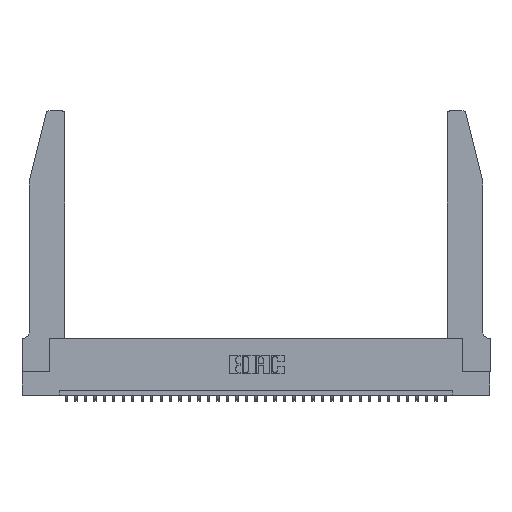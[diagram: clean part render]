
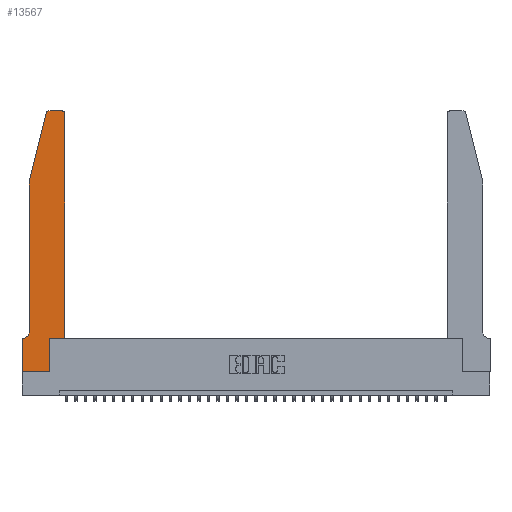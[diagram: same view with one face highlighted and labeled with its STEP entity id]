
A CAD part, top view. The second image highlights one B-rep face of the part: STEP entity #13567.
In plain terms, the highlighted planar face has unit normal (0, 0, 1).
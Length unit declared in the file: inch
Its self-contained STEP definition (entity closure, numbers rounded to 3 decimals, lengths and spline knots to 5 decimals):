
#1578 = CIRCLE ( 'NONE', #30571, 0.07 ) ;
#1940 = VERTEX_POINT ( 'NONE', #26378 ) ;
#2001 = VECTOR ( 'NONE', #25602, 39.37008 ) ;
#2040 = DIRECTION ( 'NONE',  ( -1., 0., 0. ) ) ;
#3359 = CARTESIAN_POINT ( 'NONE',  ( 0.0755, 0.35, 0.37 ) ) ;
#3652 = CARTESIAN_POINT ( 'NONE',  ( 0.0755, 2., 0.37 ) ) ;
#4504 = VERTEX_POINT ( 'NONE', #26337 ) ;
#4756 = FACE_OUTER_BOUND ( 'NONE', #33299, .T. ) ;
#4807 = DIRECTION ( 'NONE',  ( 0., -1., 0. ) ) ;
#4851 = EDGE_CURVE ( 'NONE', #34285, #14221, #1578, .T. ) ;
#5038 = CARTESIAN_POINT ( 'NONE',  ( 0.2865, 0., 0.37 ) ) ;
#5318 = DIRECTION ( 'NONE',  ( 1., 0., 0. ) ) ;
#5540 = CIRCLE ( 'NONE', #31181, 0.03 ) ;
#5613 = CARTESIAN_POINT ( 'NONE',  ( 0.4205, 2.72, 0.37 ) ) ;
#5656 = VERTEX_POINT ( 'NONE', #18806 ) ;
#6064 = CARTESIAN_POINT ( 'NONE',  ( 0.4205, 2.75, 0.37 ) ) ;
#6133 = LINE ( 'NONE', #14426, #34694 ) ;
#6441 = VERTEX_POINT ( 'NONE', #11269 ) ;
#6452 = PLANE ( 'NONE',  #11961 ) ;
#6945 = EDGE_CURVE ( 'NONE', #1940, #31079, #32196, .T. ) ;
#6946 = LINE ( 'NONE', #15786, #14725 ) ;
#8087 = CARTESIAN_POINT ( 'NONE',  ( 0.2865, 0.35, 0.37 ) ) ;
#8233 = DIRECTION ( 'NONE',  ( 0., 1., 0. ) ) ;
#8381 = VECTOR ( 'NONE', #14145, 39.37008 ) ;
#8932 = EDGE_CURVE ( 'NONE', #31079, #4504, #35767, .T. ) ;
#9596 = EDGE_CURVE ( 'NONE', #14956, #16429, #27483, .T. ) ;
#9905 = VERTEX_POINT ( 'NONE', #13331 ) ;
#11269 = CARTESIAN_POINT ( 'NONE',  ( 0., 0.35, 0.37 ) ) ;
#11312 = LINE ( 'NONE', #28334, #33819 ) ;
#11961 = AXIS2_PLACEMENT_3D ( 'NONE', #23105, #12097, #31489 ) ;
#11987 = DIRECTION ( 'NONE',  ( -0.239, -0.971, 0. ) ) ;
#12097 = DIRECTION ( 'NONE',  ( 0., 0., 1. ) ) ;
#12494 = DIRECTION ( 'NONE',  ( 1., 0., 0. ) ) ;
#13331 = CARTESIAN_POINT ( 'NONE',  ( 0.4505, 2.72, 0.37 ) ) ;
#13567 = ADVANCED_FACE ( 'NONE', ( #4756 ), #6452, .T. ) ;
#14145 = DIRECTION ( 'NONE',  ( 1., 0., 0. ) ) ;
#14221 = VERTEX_POINT ( 'NONE', #35136 ) ;
#14426 = CARTESIAN_POINT ( 'NONE',  ( 0.4505, 0.35, 0.37 ) ) ;
#14725 = VECTOR ( 'NONE', #8233, 39.37008 ) ;
#14874 = AXIS2_PLACEMENT_3D ( 'NONE', #5613, #24961, #25437 ) ;
#14956 = VERTEX_POINT ( 'NONE', #6064 ) ;
#15487 = CARTESIAN_POINT ( 'NONE',  ( 0.0055, 0.42, 0.37 ) ) ;
#15633 = EDGE_CURVE ( 'NONE', #14221, #6441, #26553, .T. ) ;
#15647 = ORIENTED_EDGE ( 'NONE', *, *, #15633, .T. ) ;
#15763 = ORIENTED_EDGE ( 'NONE', *, *, #18955, .T. ) ;
#15786 = CARTESIAN_POINT ( 'NONE',  ( 0.4505, 0.35, 0.37 ) ) ;
#16429 = VERTEX_POINT ( 'NONE', #25881 ) ;
#16665 = ORIENTED_EDGE ( 'NONE', *, *, #4851, .T. ) ;
#17924 = ORIENTED_EDGE ( 'NONE', *, *, #21050, .T. ) ;
#18806 = CARTESIAN_POINT ( 'NONE',  ( 0.4505, 0.35, 0.37 ) ) ;
#18955 = EDGE_CURVE ( 'NONE', #16429, #19744, #5540, .T. ) ;
#19340 = VECTOR ( 'NONE', #31335, 39.37008 ) ;
#19460 = ORIENTED_EDGE ( 'NONE', *, *, #6945, .T. ) ;
#19566 = VECTOR ( 'NONE', #22664, 39.37008 ) ;
#19744 = VERTEX_POINT ( 'NONE', #33013 ) ;
#20130 = ORIENTED_EDGE ( 'NONE', *, *, #29502, .T. ) ;
#20950 = DIRECTION ( 'NONE',  ( 0., 0., -1. ) ) ;
#20982 = ORIENTED_EDGE ( 'NONE', *, *, #32596, .T. ) ;
#21050 = EDGE_CURVE ( 'NONE', #25322, #34285, #34142, .T. ) ;
#22664 = DIRECTION ( 'NONE',  ( -1., 0., 0. ) ) ;
#23105 = CARTESIAN_POINT ( 'NONE',  ( 0., 0.35, 0.37 ) ) ;
#23818 = ORIENTED_EDGE ( 'NONE', *, *, #29872, .T. ) ;
#24061 = LINE ( 'NONE', #27179, #25353 ) ;
#24082 = VECTOR ( 'NONE', #28851, 39.37008 ) ;
#24961 = DIRECTION ( 'NONE',  ( 0., 0., 1. ) ) ;
#25322 = VERTEX_POINT ( 'NONE', #28209 ) ;
#25353 = VECTOR ( 'NONE', #4807, 39.37008 ) ;
#25356 = ORIENTED_EDGE ( 'NONE', *, *, #9596, .T. ) ;
#25437 = DIRECTION ( 'NONE',  ( 1., 0., 0. ) ) ;
#25602 = DIRECTION ( 'NONE',  ( -1., 0., 0. ) ) ;
#25881 = CARTESIAN_POINT ( 'NONE',  ( 0.284, 2.75, 0.37 ) ) ;
#26053 = EDGE_CURVE ( 'NONE', #4504, #5656, #6133, .T. ) ;
#26336 = CARTESIAN_POINT ( 'NONE',  ( 0.0755, 0.42, 0.37 ) ) ;
#26337 = CARTESIAN_POINT ( 'NONE',  ( 0.2865, 0.35, 0.37 ) ) ;
#26378 = CARTESIAN_POINT ( 'NONE',  ( 0., 0., 0.37 ) ) ;
#26553 = LINE ( 'NONE', #3359, #19566 ) ;
#26958 = CIRCLE ( 'NONE', #14874, 0.03 ) ;
#27179 = CARTESIAN_POINT ( 'NONE',  ( 0., 0., 0.37 ) ) ;
#27220 = DIRECTION ( 'NONE',  ( 0., 0., 1. ) ) ;
#27483 = LINE ( 'NONE', #30934, #2001 ) ;
#28209 = CARTESIAN_POINT ( 'NONE',  ( 0.0755, 2., 0.37 ) ) ;
#28225 = EDGE_CURVE ( 'NONE', #9905, #14956, #26958, .T. ) ;
#28282 = ORIENTED_EDGE ( 'NONE', *, *, #26053, .T. ) ;
#28334 = CARTESIAN_POINT ( 'NONE',  ( 0.0755, 2., 0.37 ) ) ;
#28851 = DIRECTION ( 'NONE',  ( 0., 1., 0. ) ) ;
#29502 = EDGE_CURVE ( 'NONE', #19744, #25322, #11312, .T. ) ;
#29872 = EDGE_CURVE ( 'NONE', #5656, #9905, #6946, .T. ) ;
#30523 = CARTESIAN_POINT ( 'NONE',  ( 0., 0., 0.37 ) ) ;
#30571 = AXIS2_PLACEMENT_3D ( 'NONE', #15487, #20950, #2040 ) ;
#30934 = CARTESIAN_POINT ( 'NONE',  ( 0.2605, 2.75, 0.37 ) ) ;
#31079 = VERTEX_POINT ( 'NONE', #5038 ) ;
#31181 = AXIS2_PLACEMENT_3D ( 'NONE', #35788, #27220, #5318 ) ;
#31335 = DIRECTION ( 'NONE',  ( 0., -1., 0. ) ) ;
#31489 = DIRECTION ( 'NONE',  ( 1., 0., 0. ) ) ;
#32196 = LINE ( 'NONE', #30523, #8381 ) ;
#32596 = EDGE_CURVE ( 'NONE', #6441, #1940, #24061, .T. ) ;
#33013 = CARTESIAN_POINT ( 'NONE',  ( 0.25487, 2.72718, 0.37 ) ) ;
#33299 = EDGE_LOOP ( 'NONE', ( #25356, #15763, #20130, #17924, #16665, #15647, #20982, #19460, #33841, #28282, #23818, #35322 ) ) ;
#33819 = VECTOR ( 'NONE', #11987, 39.37008 ) ;
#33841 = ORIENTED_EDGE ( 'NONE', *, *, #8932, .T. ) ;
#34142 = LINE ( 'NONE', #3652, #19340 ) ;
#34285 = VERTEX_POINT ( 'NONE', #26336 ) ;
#34694 = VECTOR ( 'NONE', #12494, 39.37008 ) ;
#35136 = CARTESIAN_POINT ( 'NONE',  ( 0.0055, 0.35, 0.37 ) ) ;
#35322 = ORIENTED_EDGE ( 'NONE', *, *, #28225, .T. ) ;
#35767 = LINE ( 'NONE', #8087, #24082 ) ;
#35788 = CARTESIAN_POINT ( 'NONE',  ( 0.284, 2.72, 0.37 ) ) ;
